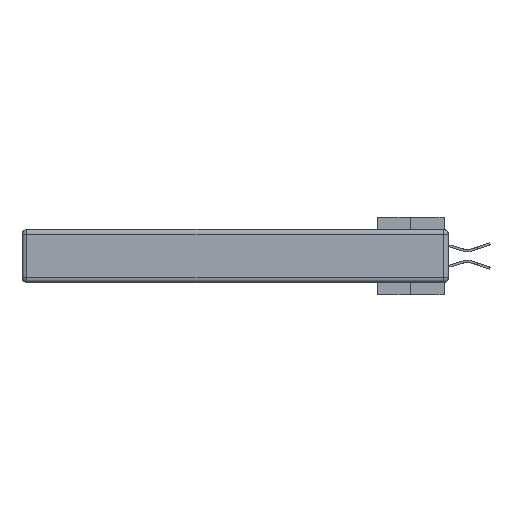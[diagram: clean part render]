
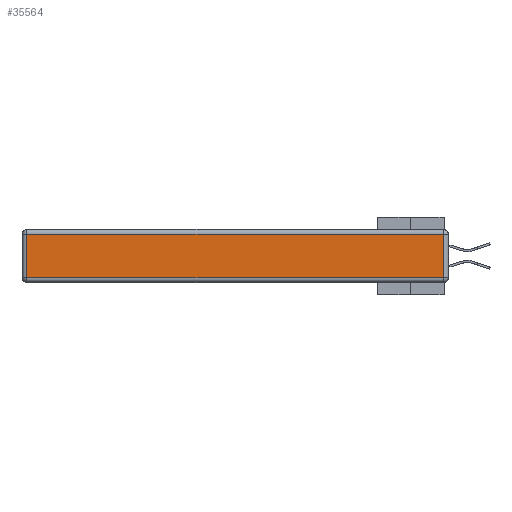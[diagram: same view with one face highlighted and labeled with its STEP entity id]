
A CAD part, left-side view. The second image highlights one B-rep face of the part: STEP entity #35564.
In plain terms, the highlighted planar face has unit normal (-1, 0, 0).
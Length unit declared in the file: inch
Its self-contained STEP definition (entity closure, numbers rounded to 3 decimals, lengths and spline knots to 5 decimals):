
#723 = DIRECTION ( 'NONE',  ( 0., 0., 1. ) ) ;
#1882 = ORIENTED_EDGE ( 'NONE', *, *, #26637, .T. ) ;
#2476 = CARTESIAN_POINT ( 'NONE',  ( 0., 0., -0.313 ) ) ;
#2739 = VECTOR ( 'NONE', #28019, 39.37008 ) ;
#5206 = ORIENTED_EDGE ( 'NONE', *, *, #12926, .T. ) ;
#7651 = ORIENTED_EDGE ( 'NONE', *, *, #24807, .T. ) ;
#8164 = LINE ( 'NONE', #2476, #15651 ) ;
#11506 = VERTEX_POINT ( 'NONE', #23927 ) ;
#11774 = ORIENTED_EDGE ( 'NONE', *, *, #27266, .T. ) ;
#12926 = EDGE_CURVE ( 'NONE', #11506, #28723, #20658, .T. ) ;
#13240 = CARTESIAN_POINT ( 'NONE',  ( 0., 2.72, -0.03 ) ) ;
#14535 = AXIS2_PLACEMENT_3D ( 'NONE', #22539, #17064, #19886 ) ;
#15616 = DIRECTION ( 'NONE',  ( 0., 0., -1. ) ) ;
#15651 = VECTOR ( 'NONE', #19393, 39.37008 ) ;
#16415 = LINE ( 'NONE', #21231, #25619 ) ;
#17064 = DIRECTION ( 'NONE',  ( -1., 0., 0. ) ) ;
#17507 = CARTESIAN_POINT ( 'NONE',  ( 0., 0.03, -0.343 ) ) ;
#19393 = DIRECTION ( 'NONE',  ( 0., -1., 0. ) ) ;
#19886 = DIRECTION ( 'NONE',  ( 0., 0., 1. ) ) ;
#20582 = CARTESIAN_POINT ( 'NONE',  ( 0., 0.03, -0.03 ) ) ;
#20658 = LINE ( 'NONE', #17507, #27218 ) ;
#21164 = LINE ( 'NONE', #30865, #2739 ) ;
#21231 = CARTESIAN_POINT ( 'NONE',  ( 0., 2.72, -0.343 ) ) ;
#22539 = CARTESIAN_POINT ( 'NONE',  ( 0., 0., -0.343 ) ) ;
#23927 = CARTESIAN_POINT ( 'NONE',  ( 0., 0.03, -0.313 ) ) ;
#24509 = CARTESIAN_POINT ( 'NONE',  ( 0., 2.72, -0.313 ) ) ;
#24807 = EDGE_CURVE ( 'NONE', #26762, #11506, #8164, .T. ) ;
#25619 = VECTOR ( 'NONE', #15616, 39.37008 ) ;
#26637 = EDGE_CURVE ( 'NONE', #26864, #26762, #16415, .T. ) ;
#26762 = VERTEX_POINT ( 'NONE', #24509 ) ;
#26864 = VERTEX_POINT ( 'NONE', #13240 ) ;
#27218 = VECTOR ( 'NONE', #723, 39.37008 ) ;
#27266 = EDGE_CURVE ( 'NONE', #28723, #26864, #21164, .T. ) ;
#28019 = DIRECTION ( 'NONE',  ( 0., 1., 0. ) ) ;
#28723 = VERTEX_POINT ( 'NONE', #20582 ) ;
#30865 = CARTESIAN_POINT ( 'NONE',  ( 0., 2.75, -0.03 ) ) ;
#31315 = PLANE ( 'NONE',  #14535 ) ;
#31553 = FACE_OUTER_BOUND ( 'NONE', #33872, .T. ) ;
#33872 = EDGE_LOOP ( 'NONE', ( #7651, #5206, #11774, #1882 ) ) ;
#35564 = ADVANCED_FACE ( 'NONE', ( #31553 ), #31315, .T. ) ;
